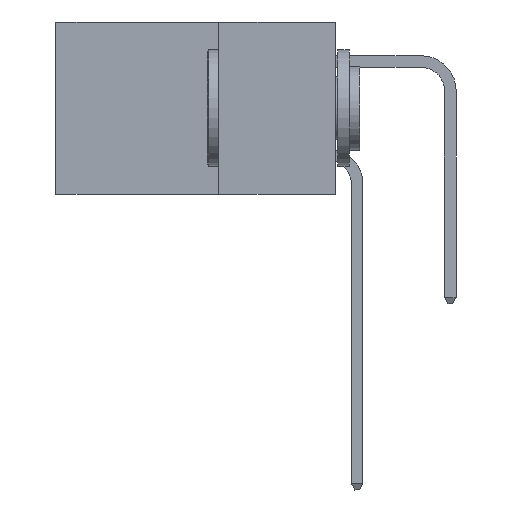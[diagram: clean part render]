
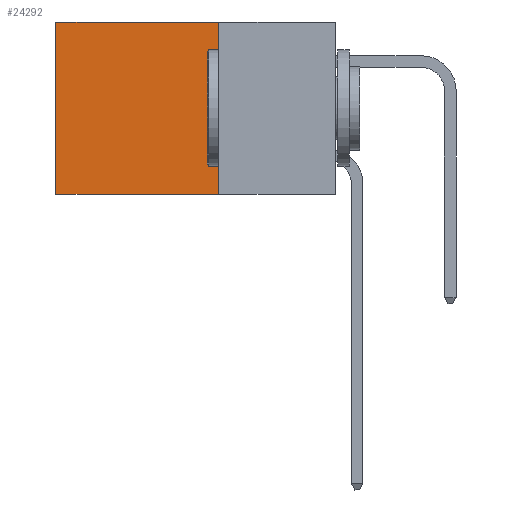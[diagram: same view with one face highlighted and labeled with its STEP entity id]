
A CAD part, left-side view. The second image highlights one B-rep face of the part: STEP entity #24292.
In plain terms, the highlighted planar face has unit normal (-1, 0, 0).
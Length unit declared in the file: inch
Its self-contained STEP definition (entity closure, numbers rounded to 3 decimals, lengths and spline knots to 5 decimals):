
#6077 = VECTOR ( 'NONE', #18053, 39.37008 ) ;
#6582 = AXIS2_PLACEMENT_3D ( 'NONE', #13903, #11327, #6590 ) ;
#6590 = DIRECTION ( 'NONE',  ( 0., 0., -1. ) ) ;
#6965 = EDGE_CURVE ( 'NONE', #15101, #28866, #8598, .T. ) ;
#7438 = CARTESIAN_POINT ( 'NONE',  ( 0.2875, 0.6, -0.37 ) ) ;
#7633 = ORIENTED_EDGE ( 'NONE', *, *, #6965, .T. ) ;
#8397 = DIRECTION ( 'NONE',  ( 0., 1., 0. ) ) ;
#8598 = LINE ( 'NONE', #12610, #21231 ) ;
#8842 = DIRECTION ( 'NONE',  ( 0., 1., 0. ) ) ;
#10005 = EDGE_CURVE ( 'NONE', #10948, #15101, #20304, .T. ) ;
#10948 = VERTEX_POINT ( 'NONE', #11720 ) ;
#11069 = ORIENTED_EDGE ( 'NONE', *, *, #10005, .T. ) ;
#11327 = DIRECTION ( 'NONE',  ( 1., 0., 0. ) ) ;
#11720 = CARTESIAN_POINT ( 'NONE',  ( 0.2875, 0.25, 0. ) ) ;
#12610 = CARTESIAN_POINT ( 'NONE',  ( 0.2875, 0.6, 0. ) ) ;
#13752 = VERTEX_POINT ( 'NONE', #24887 ) ;
#13903 = CARTESIAN_POINT ( 'NONE',  ( 0.2875, 0.25, 0. ) ) ;
#15101 = VERTEX_POINT ( 'NONE', #16102 ) ;
#15484 = EDGE_CURVE ( 'NONE', #10948, #13752, #16807, .T. ) ;
#16102 = CARTESIAN_POINT ( 'NONE',  ( 0.2875, 0.6, 0. ) ) ;
#16807 = LINE ( 'NONE', #28159, #6077 ) ;
#18053 = DIRECTION ( 'NONE',  ( 0., 0., -1. ) ) ;
#18842 = LINE ( 'NONE', #27892, #29991 ) ;
#19567 = ORIENTED_EDGE ( 'NONE', *, *, #31133, .F. ) ;
#20297 = ORIENTED_EDGE ( 'NONE', *, *, #15484, .F. ) ;
#20304 = LINE ( 'NONE', #31393, #27478 ) ;
#21231 = VECTOR ( 'NONE', #22388, 39.37008 ) ;
#22388 = DIRECTION ( 'NONE',  ( 0., 0., -1. ) ) ;
#24292 = ADVANCED_FACE ( 'NONE', ( #31264 ), #26359, .F. ) ;
#24887 = CARTESIAN_POINT ( 'NONE',  ( 0.2875, 0.25, -0.37 ) ) ;
#24978 = EDGE_LOOP ( 'NONE', ( #7633, #19567, #20297, #11069 ) ) ;
#26359 = PLANE ( 'NONE',  #6582 ) ;
#27478 = VECTOR ( 'NONE', #8842, 39.37008 ) ;
#27892 = CARTESIAN_POINT ( 'NONE',  ( 0.2875, 0.25, -0.37 ) ) ;
#28159 = CARTESIAN_POINT ( 'NONE',  ( 0.2875, 0.25, 0. ) ) ;
#28866 = VERTEX_POINT ( 'NONE', #7438 ) ;
#29991 = VECTOR ( 'NONE', #8397, 39.37008 ) ;
#31133 = EDGE_CURVE ( 'NONE', #13752, #28866, #18842, .T. ) ;
#31264 = FACE_OUTER_BOUND ( 'NONE', #24978, .T. ) ;
#31393 = CARTESIAN_POINT ( 'NONE',  ( 0.2875, 0.25, 0. ) ) ;
